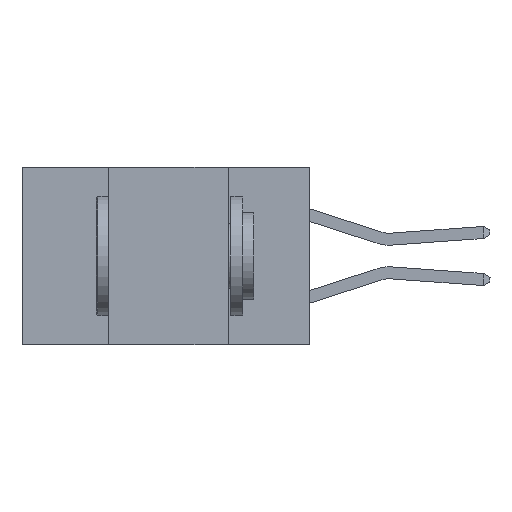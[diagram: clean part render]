
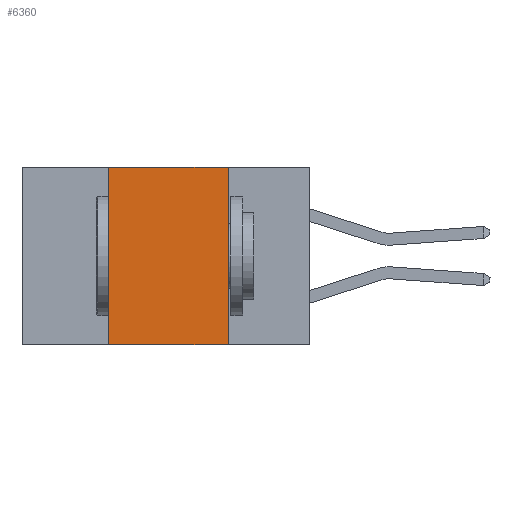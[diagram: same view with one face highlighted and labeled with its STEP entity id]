
A CAD part, left-side view. The second image highlights one B-rep face of the part: STEP entity #6360.
In plain terms, the highlighted planar face has unit normal (-1, 0, 0).
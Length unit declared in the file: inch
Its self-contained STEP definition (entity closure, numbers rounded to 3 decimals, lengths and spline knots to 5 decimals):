
#1091 = CARTESIAN_POINT ( 'NONE',  ( 0., 0.6, 0. ) ) ;
#1157 = DIRECTION ( 'NONE',  ( 0., -1., 0. ) ) ;
#2260 = VERTEX_POINT ( 'NONE', #11333 ) ;
#2570 = CARTESIAN_POINT ( 'NONE',  ( 0., 0.42, -0.37 ) ) ;
#2641 = VERTEX_POINT ( 'NONE', #7184 ) ;
#2661 = EDGE_CURVE ( 'NONE', #18255, #2260, #17229, .T. ) ;
#3072 = LINE ( 'NONE', #1091, #19961 ) ;
#3311 = LINE ( 'NONE', #15545, #17125 ) ;
#4195 = EDGE_CURVE ( 'NONE', #2641, #2260, #16434, .T. ) ;
#5404 = CARTESIAN_POINT ( 'NONE',  ( 0., 0.6, -0.37 ) ) ;
#5730 = CARTESIAN_POINT ( 'NONE',  ( 0., 0.17, 0. ) ) ;
#5981 = EDGE_LOOP ( 'NONE', ( #15826, #15850, #11314, #14463 ) ) ;
#6360 = ADVANCED_FACE ( 'NONE', ( #18192 ), #8269, .F. ) ;
#7184 = CARTESIAN_POINT ( 'NONE',  ( 0., 0.17, 0. ) ) ;
#7196 = EDGE_CURVE ( 'NONE', #10393, #2641, #3072, .T. ) ;
#7620 = EDGE_CURVE ( 'NONE', #18255, #10393, #3311, .T. ) ;
#8269 = PLANE ( 'NONE',  #20599 ) ;
#8795 = DIRECTION ( 'NONE',  ( 0., -1., 0. ) ) ;
#8909 = DIRECTION ( 'NONE',  ( 0., 0., -1. ) ) ;
#10393 = VERTEX_POINT ( 'NONE', #14978 ) ;
#10565 = VECTOR ( 'NONE', #8795, 39.37008 ) ;
#11314 = ORIENTED_EDGE ( 'NONE', *, *, #7620, .F. ) ;
#11333 = CARTESIAN_POINT ( 'NONE',  ( 0., 0.17, -0.37 ) ) ;
#12334 = DIRECTION ( 'NONE',  ( 0., 0., 1. ) ) ;
#14463 = ORIENTED_EDGE ( 'NONE', *, *, #2661, .T. ) ;
#14978 = CARTESIAN_POINT ( 'NONE',  ( 0., 0.42, 0. ) ) ;
#15417 = VECTOR ( 'NONE', #8909, 39.37008 ) ;
#15545 = CARTESIAN_POINT ( 'NONE',  ( 0., 0.42, 0. ) ) ;
#15826 = ORIENTED_EDGE ( 'NONE', *, *, #4195, .F. ) ;
#15850 = ORIENTED_EDGE ( 'NONE', *, *, #7196, .F. ) ;
#16434 = LINE ( 'NONE', #5730, #15417 ) ;
#17125 = VECTOR ( 'NONE', #12334, 39.37008 ) ;
#17229 = LINE ( 'NONE', #5404, #10565 ) ;
#17789 = DIRECTION ( 'NONE',  ( 1., 0., 0. ) ) ;
#18192 = FACE_OUTER_BOUND ( 'NONE', #5981, .T. ) ;
#18255 = VERTEX_POINT ( 'NONE', #2570 ) ;
#19432 = DIRECTION ( 'NONE',  ( 0., 0., -1. ) ) ;
#19576 = CARTESIAN_POINT ( 'NONE',  ( 0., 0.6, 0. ) ) ;
#19961 = VECTOR ( 'NONE', #1157, 39.37008 ) ;
#20599 = AXIS2_PLACEMENT_3D ( 'NONE', #19576, #17789, #19432 ) ;
